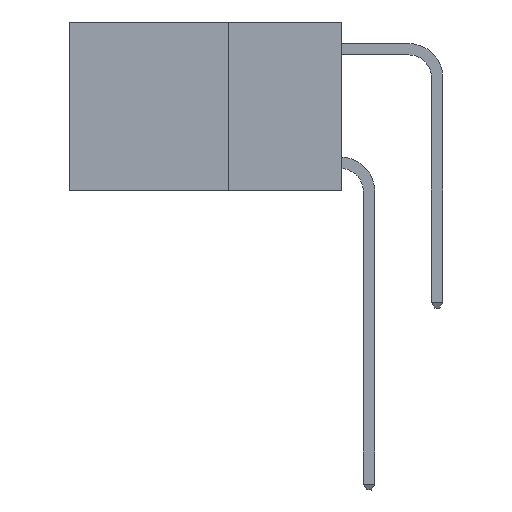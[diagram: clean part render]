
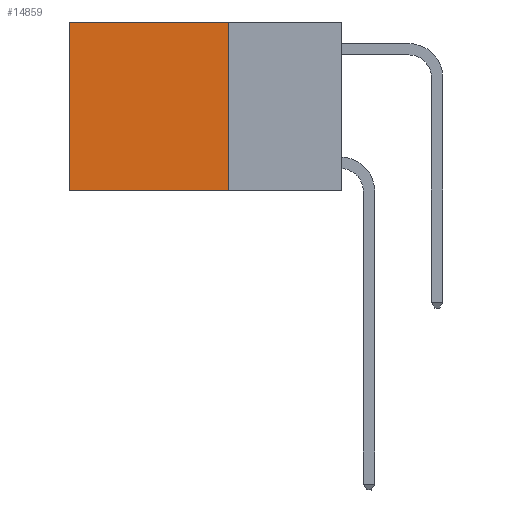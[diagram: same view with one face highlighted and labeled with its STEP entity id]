
A CAD part, left-side view. The second image highlights one B-rep face of the part: STEP entity #14859.
In plain terms, the highlighted planar face has unit normal (-1, 0, 0).
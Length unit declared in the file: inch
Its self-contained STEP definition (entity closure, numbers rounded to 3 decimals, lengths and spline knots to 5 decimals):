
#355 = CARTESIAN_POINT ( 'NONE',  ( 0.2625, 0.25, 0. ) ) ;
#475 = LINE ( 'NONE', #15228, #8398 ) ;
#910 = CARTESIAN_POINT ( 'NONE',  ( 0.2625, 0.25, -0.37 ) ) ;
#999 = DIRECTION ( 'NONE',  ( 0., 1., 0. ) ) ;
#1824 = VERTEX_POINT ( 'NONE', #910 ) ;
#2639 = CARTESIAN_POINT ( 'NONE',  ( 0.2625, 0.25, -0.37 ) ) ;
#3657 = CARTESIAN_POINT ( 'NONE',  ( 0.2625, 0.6, 0. ) ) ;
#3926 = EDGE_LOOP ( 'NONE', ( #18000, #8465, #16949, #10760 ) ) ;
#4938 = FACE_OUTER_BOUND ( 'NONE', #3926, .T. ) ;
#5232 = LINE ( 'NONE', #5743, #8921 ) ;
#5743 = CARTESIAN_POINT ( 'NONE',  ( 0.2625, 0.25, 0. ) ) ;
#6744 = PLANE ( 'NONE',  #17500 ) ;
#7746 = VERTEX_POINT ( 'NONE', #3657 ) ;
#7896 = EDGE_CURVE ( 'NONE', #7746, #9273, #8798, .T. ) ;
#8307 = DIRECTION ( 'NONE',  ( 1., 0., 0. ) ) ;
#8398 = VECTOR ( 'NONE', #999, 39.37008 ) ;
#8465 = ORIENTED_EDGE ( 'NONE', *, *, #17375, .F. ) ;
#8798 = LINE ( 'NONE', #10445, #13057 ) ;
#8921 = VECTOR ( 'NONE', #15231, 39.37008 ) ;
#9273 = VERTEX_POINT ( 'NONE', #15405 ) ;
#10445 = CARTESIAN_POINT ( 'NONE',  ( 0.2625, 0.6, 0. ) ) ;
#10760 = ORIENTED_EDGE ( 'NONE', *, *, #15367, .T. ) ;
#11489 = CARTESIAN_POINT ( 'NONE',  ( 0.2625, 0.25, 0. ) ) ;
#11950 = VECTOR ( 'NONE', #18512, 39.37008 ) ;
#13057 = VECTOR ( 'NONE', #19877, 39.37008 ) ;
#13712 = EDGE_CURVE ( 'NONE', #18591, #1824, #5232, .T. ) ;
#14859 = ADVANCED_FACE ( 'NONE', ( #4938 ), #6744, .F. ) ;
#15228 = CARTESIAN_POINT ( 'NONE',  ( 0.2625, 0.25, 0. ) ) ;
#15231 = DIRECTION ( 'NONE',  ( 0., 0., -1. ) ) ;
#15367 = EDGE_CURVE ( 'NONE', #18591, #7746, #475, .T. ) ;
#15405 = CARTESIAN_POINT ( 'NONE',  ( 0.2625, 0.6, -0.37 ) ) ;
#16122 = LINE ( 'NONE', #2639, #11950 ) ;
#16949 = ORIENTED_EDGE ( 'NONE', *, *, #13712, .F. ) ;
#17375 = EDGE_CURVE ( 'NONE', #1824, #9273, #16122, .T. ) ;
#17500 = AXIS2_PLACEMENT_3D ( 'NONE', #355, #8307, #19379 ) ;
#18000 = ORIENTED_EDGE ( 'NONE', *, *, #7896, .T. ) ;
#18512 = DIRECTION ( 'NONE',  ( 0., 1., 0. ) ) ;
#18591 = VERTEX_POINT ( 'NONE', #11489 ) ;
#19379 = DIRECTION ( 'NONE',  ( 0., 0., -1. ) ) ;
#19877 = DIRECTION ( 'NONE',  ( 0., 0., -1. ) ) ;
